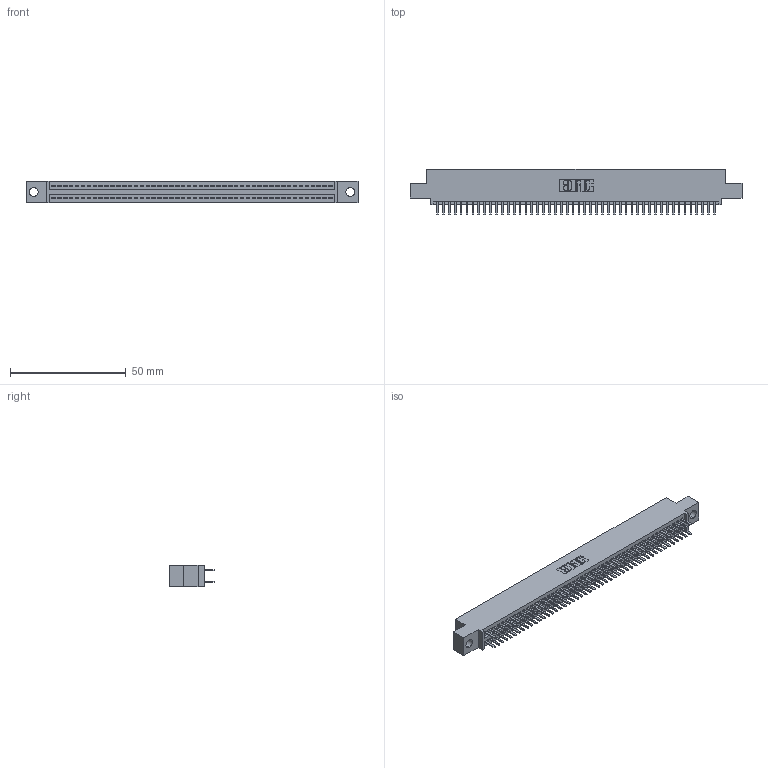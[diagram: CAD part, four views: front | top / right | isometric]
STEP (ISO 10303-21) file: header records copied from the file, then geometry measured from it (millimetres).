
FILE_DESCRIPTION (( 'STEP AP203' ), '1' );
FILE_NAME ('345-096-520-504.STEP', '2021-05-20T16:55:17', ( '' ), ( '' ), 'SwSTEP 2.0', 'SolidWorks 2020', '' );
FILE_SCHEMA (( 'CONFIG_CONTROL_DESIGN' ));
Length unit declared in the file: inch
Products named in the file (3): 345-292-001_345-293-120; 345 Part_0.110 Offset - 0.156 Dia-TI; 345-096-520-504
Assembly tree (97 placements, depth 2):
  345-096-520-504
    345 Part_0.110 Offset - 0.156 Dia-TI
    345-292-001_345-293-120  x96
Bounding box: 143.13 x 19.68 x 9.4 mm (x, y, z)
Volume: 13737.9 mm3; surface area: 20277.8 mm2
Topology: 97 solids, 97 shells, 5328 faces, 15461 edges, 10050 vertices
Faces by surface type: plane 3458, cylinder 1870
Entity records: 37519 total; most frequent: CARTESIAN_POINT 6302, ORIENTED_EDGE 6222, DIRECTION 5535, EDGE_CURVE 3111, VECTOR 2783, LINE 2783, VERTEX_POINT 2070, AXIS2_PLACEMENT_3D 1376
